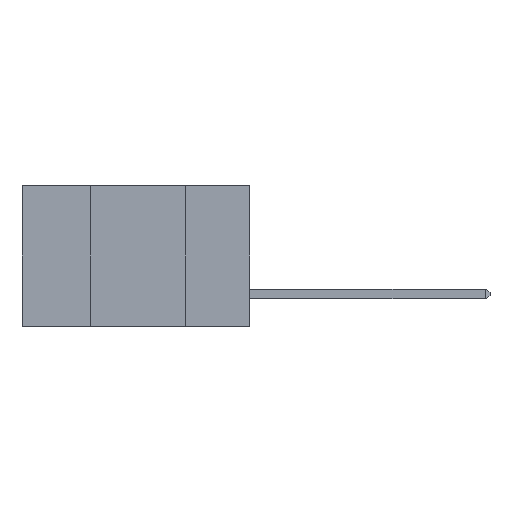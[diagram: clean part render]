
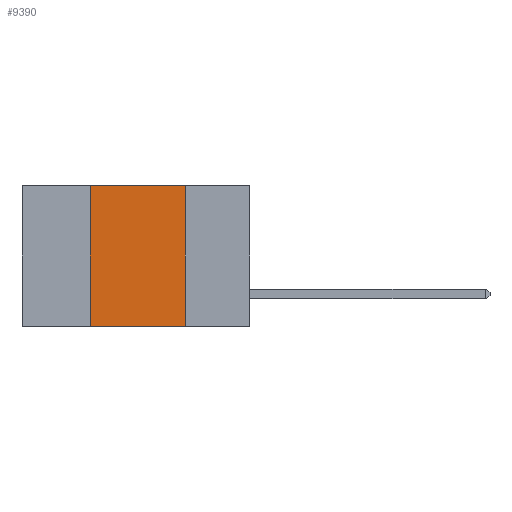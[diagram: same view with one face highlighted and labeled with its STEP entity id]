
A CAD part, left-side view. The second image highlights one B-rep face of the part: STEP entity #9390.
In plain terms, the highlighted planar face has unit normal (-1, 0, 0).
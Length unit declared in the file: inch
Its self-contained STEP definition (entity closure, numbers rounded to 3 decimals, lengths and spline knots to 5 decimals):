
#171 = VECTOR ( 'NONE', #1961, 39.37008 ) ;
#586 = FACE_OUTER_BOUND ( 'NONE', #19656, .T. ) ;
#889 = CARTESIAN_POINT ( 'NONE',  ( 0., 0.42, 0. ) ) ;
#1108 = AXIS2_PLACEMENT_3D ( 'NONE', #17697, #19126, #10190 ) ;
#1425 = VECTOR ( 'NONE', #1584, 39.37008 ) ;
#1584 = DIRECTION ( 'NONE',  ( 0., 0., 1. ) ) ;
#1961 = DIRECTION ( 'NONE',  ( 0., -1., 0. ) ) ;
#2806 = VERTEX_POINT ( 'NONE', #2941 ) ;
#2941 = CARTESIAN_POINT ( 'NONE',  ( 0., 0.42, 0. ) ) ;
#2980 = CARTESIAN_POINT ( 'NONE',  ( 0., 0.17, 0. ) ) ;
#3182 = CARTESIAN_POINT ( 'NONE',  ( 0., 0.42, -0.37 ) ) ;
#4672 = DIRECTION ( 'NONE',  ( 0., 0., -1. ) ) ;
#5126 = LINE ( 'NONE', #17127, #16314 ) ;
#5295 = CARTESIAN_POINT ( 'NONE',  ( 0., 0.6, 0. ) ) ;
#5597 = EDGE_CURVE ( 'NONE', #13027, #2806, #9936, .T. ) ;
#6391 = ORIENTED_EDGE ( 'NONE', *, *, #17792, .F. ) ;
#6417 = CARTESIAN_POINT ( 'NONE',  ( 0., 0.17, -0.37 ) ) ;
#9390 = ADVANCED_FACE ( 'NONE', ( #586 ), #16218, .F. ) ;
#9514 = VERTEX_POINT ( 'NONE', #19371 ) ;
#9650 = LINE ( 'NONE', #2980, #17245 ) ;
#9936 = LINE ( 'NONE', #889, #1425 ) ;
#10190 = DIRECTION ( 'NONE',  ( 0., 0., -1. ) ) ;
#11131 = DIRECTION ( 'NONE',  ( 0., -1., 0. ) ) ;
#11425 = ORIENTED_EDGE ( 'NONE', *, *, #5597, .F. ) ;
#11888 = ORIENTED_EDGE ( 'NONE', *, *, #17453, .T. ) ;
#13027 = VERTEX_POINT ( 'NONE', #3182 ) ;
#15788 = EDGE_CURVE ( 'NONE', #2806, #9514, #17336, .T. ) ;
#16218 = PLANE ( 'NONE',  #1108 ) ;
#16314 = VECTOR ( 'NONE', #11131, 39.37008 ) ;
#16785 = VERTEX_POINT ( 'NONE', #6417 ) ;
#17127 = CARTESIAN_POINT ( 'NONE',  ( 0., 0.6, -0.37 ) ) ;
#17245 = VECTOR ( 'NONE', #4672, 39.37008 ) ;
#17336 = LINE ( 'NONE', #5295, #171 ) ;
#17453 = EDGE_CURVE ( 'NONE', #13027, #16785, #5126, .T. ) ;
#17697 = CARTESIAN_POINT ( 'NONE',  ( 0., 0.6, 0. ) ) ;
#17792 = EDGE_CURVE ( 'NONE', #9514, #16785, #9650, .T. ) ;
#18846 = ORIENTED_EDGE ( 'NONE', *, *, #15788, .F. ) ;
#19126 = DIRECTION ( 'NONE',  ( 1., 0., 0. ) ) ;
#19371 = CARTESIAN_POINT ( 'NONE',  ( 0., 0.17, 0. ) ) ;
#19656 = EDGE_LOOP ( 'NONE', ( #6391, #18846, #11425, #11888 ) ) ;
